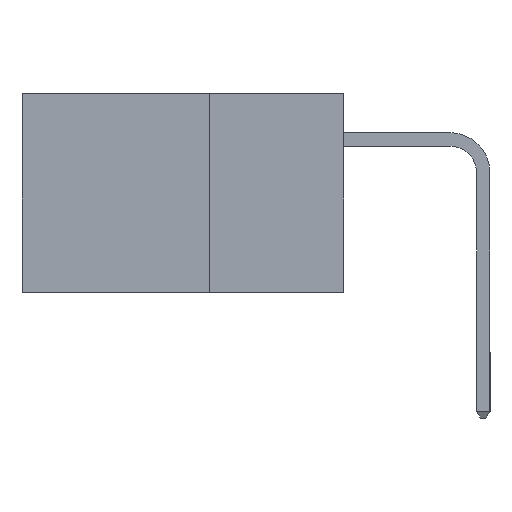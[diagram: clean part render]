
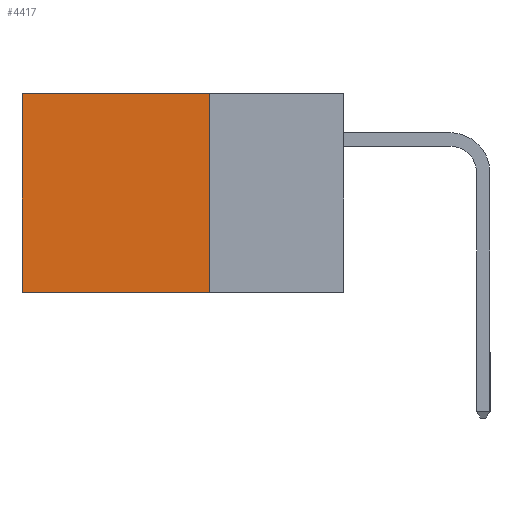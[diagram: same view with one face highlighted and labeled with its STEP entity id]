
A CAD part, left-side view. The second image highlights one B-rep face of the part: STEP entity #4417.
In plain terms, the highlighted planar face has unit normal (-1, 0, 0).
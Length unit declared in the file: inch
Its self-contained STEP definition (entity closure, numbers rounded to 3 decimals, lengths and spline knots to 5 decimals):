
#49 = DIRECTION ( 'NONE',  ( 0., 0., -1. ) ) ;
#60 = CARTESIAN_POINT ( 'NONE',  ( 0.2615, 0.6, 0. ) ) ;
#771 = CARTESIAN_POINT ( 'NONE',  ( 0.2615, 0.25, -0.37 ) ) ;
#1206 = VERTEX_POINT ( 'NONE', #6272 ) ;
#1650 = VECTOR ( 'NONE', #9926, 39.37008 ) ;
#1849 = EDGE_CURVE ( 'NONE', #4006, #10012, #3517, .T. ) ;
#2137 = EDGE_CURVE ( 'NONE', #1206, #2883, #10829, .T. ) ;
#2883 = VERTEX_POINT ( 'NONE', #3102 ) ;
#3102 = CARTESIAN_POINT ( 'NONE',  ( 0.2615, 0.25, -0.37 ) ) ;
#3199 = PLANE ( 'NONE',  #9105 ) ;
#3517 = LINE ( 'NONE', #4602, #5501 ) ;
#3863 = ORIENTED_EDGE ( 'NONE', *, *, #8144, .T. ) ;
#4006 = VERTEX_POINT ( 'NONE', #60 ) ;
#4196 = VECTOR ( 'NONE', #6120, 39.37008 ) ;
#4270 = CARTESIAN_POINT ( 'NONE',  ( 0.2615, 0.25, 0. ) ) ;
#4417 = ADVANCED_FACE ( 'NONE', ( #5871 ), #3199, .F. ) ;
#4602 = CARTESIAN_POINT ( 'NONE',  ( 0.2615, 0.6, -0.37 ) ) ;
#4671 = ORIENTED_EDGE ( 'NONE', *, *, #1849, .T. ) ;
#4914 = CARTESIAN_POINT ( 'NONE',  ( 0.2615, 0.25, -0.37 ) ) ;
#4964 = VECTOR ( 'NONE', #7507, 39.37008 ) ;
#5072 = LINE ( 'NONE', #4270, #4196 ) ;
#5357 = DIRECTION ( 'NONE',  ( 0., 0., -1. ) ) ;
#5501 = VECTOR ( 'NONE', #5357, 39.37008 ) ;
#5629 = CARTESIAN_POINT ( 'NONE',  ( 0.2615, 0.25, -0.37 ) ) ;
#5818 = DIRECTION ( 'NONE',  ( 1., 0., 0. ) ) ;
#5871 = FACE_OUTER_BOUND ( 'NONE', #9158, .T. ) ;
#6120 = DIRECTION ( 'NONE',  ( 0., 1., 0. ) ) ;
#6272 = CARTESIAN_POINT ( 'NONE',  ( 0.2615, 0.25, 0. ) ) ;
#6592 = LINE ( 'NONE', #5629, #1650 ) ;
#6972 = ORIENTED_EDGE ( 'NONE', *, *, #2137, .F. ) ;
#7507 = DIRECTION ( 'NONE',  ( 0., 0., -1. ) ) ;
#8144 = EDGE_CURVE ( 'NONE', #1206, #4006, #5072, .T. ) ;
#8389 = EDGE_CURVE ( 'NONE', #2883, #10012, #6592, .T. ) ;
#8401 = ORIENTED_EDGE ( 'NONE', *, *, #8389, .F. ) ;
#8496 = CARTESIAN_POINT ( 'NONE',  ( 0.2615, 0.6, -0.37 ) ) ;
#9105 = AXIS2_PLACEMENT_3D ( 'NONE', #771, #5818, #49 ) ;
#9158 = EDGE_LOOP ( 'NONE', ( #4671, #8401, #6972, #3863 ) ) ;
#9926 = DIRECTION ( 'NONE',  ( 0., 1., 0. ) ) ;
#10012 = VERTEX_POINT ( 'NONE', #8496 ) ;
#10829 = LINE ( 'NONE', #4914, #4964 ) ;
